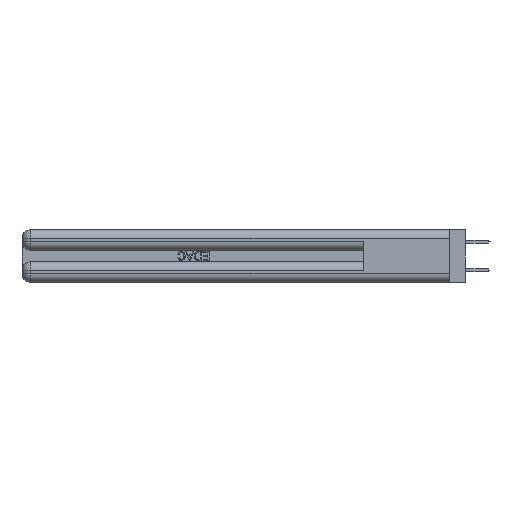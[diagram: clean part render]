
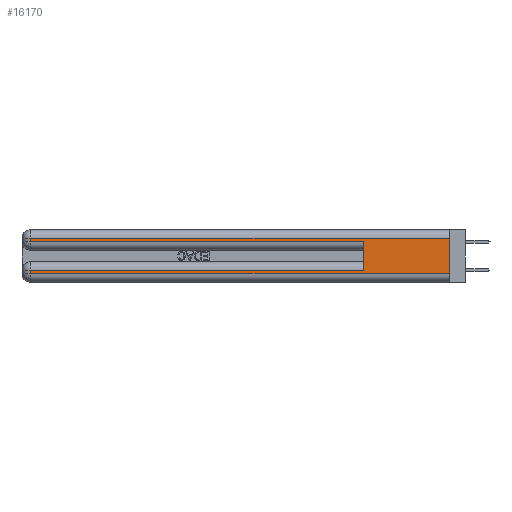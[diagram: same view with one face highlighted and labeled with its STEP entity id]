
A CAD part, left-side view. The second image highlights one B-rep face of the part: STEP entity #16170.
In plain terms, the highlighted planar face has unit normal (-1, 0, 0).
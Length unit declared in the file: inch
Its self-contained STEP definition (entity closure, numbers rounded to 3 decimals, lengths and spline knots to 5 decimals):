
#339 = LINE ( 'NONE', #20543, #41189 ) ;
#1354 = CARTESIAN_POINT ( 'NONE',  ( 0., 0., 0.37 ) ) ;
#1641 = CARTESIAN_POINT ( 'NONE',  ( 0., 0., 0.085 ) ) ;
#1700 = DIRECTION ( 'NONE',  ( 0., 1., 0. ) ) ;
#1888 = VERTEX_POINT ( 'NONE', #38396 ) ;
#2108 = CARTESIAN_POINT ( 'NONE',  ( 0., 0.6, 0.285 ) ) ;
#3639 = VECTOR ( 'NONE', #16735, 39.37008 ) ;
#3696 = ORIENTED_EDGE ( 'NONE', *, *, #32744, .T. ) ;
#5223 = PLANE ( 'NONE',  #26252 ) ;
#5788 = ORIENTED_EDGE ( 'NONE', *, *, #32458, .F. ) ;
#5829 = CARTESIAN_POINT ( 'NONE',  ( 0., 2.94, 0.37 ) ) ;
#6495 = LINE ( 'NONE', #22596, #42799 ) ;
#7034 = EDGE_CURVE ( 'NONE', #12812, #34751, #10505, .T. ) ;
#7038 = CARTESIAN_POINT ( 'NONE',  ( 0., 0., 0.285 ) ) ;
#7612 = CARTESIAN_POINT ( 'NONE',  ( 0., 0., 0.06 ) ) ;
#8259 = EDGE_CURVE ( 'NONE', #1888, #8412, #25740, .T. ) ;
#8412 = VERTEX_POINT ( 'NONE', #2108 ) ;
#9138 = EDGE_CURVE ( 'NONE', #43977, #24102, #6495, .T. ) ;
#9489 = EDGE_LOOP ( 'NONE', ( #5788, #41801, #23068, #21914, #40331, #38825, #3696, #20488 ) ) ;
#9885 = DIRECTION ( 'NONE',  ( 0., 0., 1. ) ) ;
#10007 = EDGE_CURVE ( 'NONE', #34927, #30797, #43347, .T. ) ;
#10125 = DIRECTION ( 'NONE',  ( 0., 0., -1. ) ) ;
#10505 = LINE ( 'NONE', #22026, #20391 ) ;
#12812 = VERTEX_POINT ( 'NONE', #35951 ) ;
#15835 = DIRECTION ( 'NONE',  ( 1., 0., 0. ) ) ;
#16170 = ADVANCED_FACE ( 'NONE', ( #34250 ), #5223, .F. ) ;
#16735 = DIRECTION ( 'NONE',  ( 0., 0., -1. ) ) ;
#19277 = CARTESIAN_POINT ( 'NONE',  ( 0., 2.94, 0.31 ) ) ;
#20019 = LINE ( 'NONE', #31399, #31054 ) ;
#20391 = VECTOR ( 'NONE', #42229, 39.37008 ) ;
#20488 = ORIENTED_EDGE ( 'NONE', *, *, #7034, .T. ) ;
#20543 = CARTESIAN_POINT ( 'NONE',  ( 0., 0., 0.37 ) ) ;
#21430 = DIRECTION ( 'NONE',  ( 0., -1., 0. ) ) ;
#21822 = CARTESIAN_POINT ( 'NONE',  ( 0., 0.6, 0.085 ) ) ;
#21914 = ORIENTED_EDGE ( 'NONE', *, *, #8259, .T. ) ;
#22026 = CARTESIAN_POINT ( 'NONE',  ( 0., 0., 0.06 ) ) ;
#22596 = CARTESIAN_POINT ( 'NONE',  ( 0., 0., 0.31 ) ) ;
#23068 = ORIENTED_EDGE ( 'NONE', *, *, #41718, .T. ) ;
#24102 = VERTEX_POINT ( 'NONE', #19277 ) ;
#25740 = LINE ( 'NONE', #7038, #42349 ) ;
#26234 = VECTOR ( 'NONE', #40919, 39.37008 ) ;
#26252 = AXIS2_PLACEMENT_3D ( 'NONE', #1354, #15835, #30030 ) ;
#27332 = LINE ( 'NONE', #5829, #3639 ) ;
#28564 = DIRECTION ( 'NONE',  ( 0., 0., -1. ) ) ;
#29059 = VECTOR ( 'NONE', #28564, 39.37008 ) ;
#30030 = DIRECTION ( 'NONE',  ( 0., 0., -1. ) ) ;
#30797 = VERTEX_POINT ( 'NONE', #36173 ) ;
#31054 = VECTOR ( 'NONE', #9885, 39.37008 ) ;
#31399 = CARTESIAN_POINT ( 'NONE',  ( 0., 0.6, 0.145 ) ) ;
#31954 = CARTESIAN_POINT ( 'NONE',  ( 0., 2.94, 0.37 ) ) ;
#32458 = EDGE_CURVE ( 'NONE', #43977, #34751, #339, .T. ) ;
#32744 = EDGE_CURVE ( 'NONE', #30797, #12812, #27332, .T. ) ;
#34250 = FACE_OUTER_BOUND ( 'NONE', #9489, .T. ) ;
#34488 = EDGE_CURVE ( 'NONE', #34927, #8412, #20019, .T. ) ;
#34751 = VERTEX_POINT ( 'NONE', #7612 ) ;
#34927 = VERTEX_POINT ( 'NONE', #21822 ) ;
#35951 = CARTESIAN_POINT ( 'NONE',  ( 0., 2.94, 0.06 ) ) ;
#36173 = CARTESIAN_POINT ( 'NONE',  ( 0., 2.94, 0.085 ) ) ;
#38396 = CARTESIAN_POINT ( 'NONE',  ( 0., 2.94, 0.285 ) ) ;
#38490 = LINE ( 'NONE', #31954, #29059 ) ;
#38825 = ORIENTED_EDGE ( 'NONE', *, *, #10007, .T. ) ;
#40331 = ORIENTED_EDGE ( 'NONE', *, *, #34488, .F. ) ;
#40919 = DIRECTION ( 'NONE',  ( 0., 1., 0. ) ) ;
#41189 = VECTOR ( 'NONE', #10125, 39.37008 ) ;
#41349 = CARTESIAN_POINT ( 'NONE',  ( 0., 0., 0.31 ) ) ;
#41718 = EDGE_CURVE ( 'NONE', #24102, #1888, #38490, .T. ) ;
#41801 = ORIENTED_EDGE ( 'NONE', *, *, #9138, .T. ) ;
#42229 = DIRECTION ( 'NONE',  ( 0., -1., 0. ) ) ;
#42349 = VECTOR ( 'NONE', #21430, 39.37008 ) ;
#42799 = VECTOR ( 'NONE', #1700, 39.37008 ) ;
#43347 = LINE ( 'NONE', #1641, #26234 ) ;
#43977 = VERTEX_POINT ( 'NONE', #41349 ) ;
